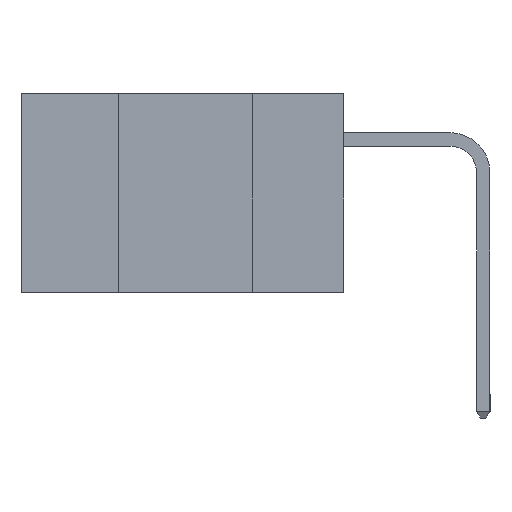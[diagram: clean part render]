
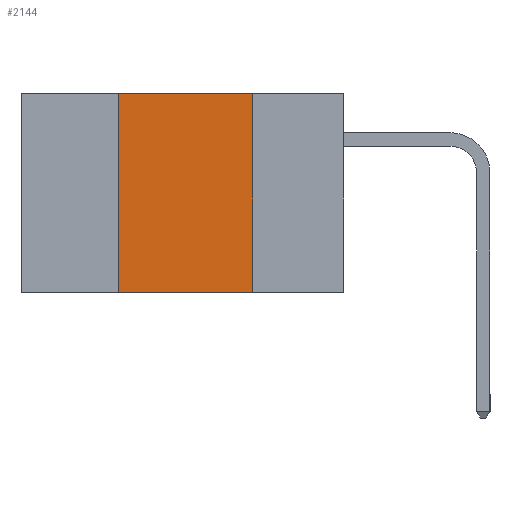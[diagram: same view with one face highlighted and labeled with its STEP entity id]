
A CAD part, left-side view. The second image highlights one B-rep face of the part: STEP entity #2144.
In plain terms, the highlighted planar face has unit normal (-1, 0, 0).
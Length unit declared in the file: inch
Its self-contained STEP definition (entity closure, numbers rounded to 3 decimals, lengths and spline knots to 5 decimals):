
#151 = EDGE_CURVE ( 'NONE', #18014, #11505, #10872, .T. ) ;
#983 = VERTEX_POINT ( 'NONE', #18293 ) ;
#1984 = CARTESIAN_POINT ( 'NONE',  ( 0., 0.17, -0.37 ) ) ;
#2144 = ADVANCED_FACE ( 'NONE', ( #19968 ), #10335, .F. ) ;
#2215 = ORIENTED_EDGE ( 'NONE', *, *, #21178, .F. ) ;
#4227 = CARTESIAN_POINT ( 'NONE',  ( 0., 0.17, -0.37 ) ) ;
#4816 = VERTEX_POINT ( 'NONE', #19660 ) ;
#5437 = VECTOR ( 'NONE', #21842, 39.37008 ) ;
#6388 = ORIENTED_EDGE ( 'NONE', *, *, #16742, .F. ) ;
#8524 = DIRECTION ( 'NONE',  ( 1., 0., 0. ) ) ;
#8575 = DIRECTION ( 'NONE',  ( 0., 0., -1. ) ) ;
#9045 = CARTESIAN_POINT ( 'NONE',  ( 0., 0.6, 0. ) ) ;
#9457 = VECTOR ( 'NONE', #14872, 39.37008 ) ;
#9510 = CARTESIAN_POINT ( 'NONE',  ( 0., 0.17, 0. ) ) ;
#9820 = AXIS2_PLACEMENT_3D ( 'NONE', #9045, #8524, #8575 ) ;
#10335 = PLANE ( 'NONE',  #9820 ) ;
#10872 = LINE ( 'NONE', #4227, #19280 ) ;
#11433 = CARTESIAN_POINT ( 'NONE',  ( 0., 0.6, 0. ) ) ;
#11505 = VERTEX_POINT ( 'NONE', #1984 ) ;
#11613 = DIRECTION ( 'NONE',  ( 0., 0., -1. ) ) ;
#13068 = ORIENTED_EDGE ( 'NONE', *, *, #151, .F. ) ;
#13365 = EDGE_CURVE ( 'NONE', #983, #11505, #13457, .T. ) ;
#13457 = LINE ( 'NONE', #20928, #21269 ) ;
#13500 = EDGE_LOOP ( 'NONE', ( #13068, #2215, #6388, #19386 ) ) ;
#13821 = LINE ( 'NONE', #21730, #5437 ) ;
#13923 = LINE ( 'NONE', #11433, #9457 ) ;
#14872 = DIRECTION ( 'NONE',  ( 0., -1., 0. ) ) ;
#16742 = EDGE_CURVE ( 'NONE', #983, #4816, #13821, .T. ) ;
#18014 = VERTEX_POINT ( 'NONE', #9510 ) ;
#18293 = CARTESIAN_POINT ( 'NONE',  ( 0., 0.42, -0.37 ) ) ;
#19280 = VECTOR ( 'NONE', #11613, 39.37008 ) ;
#19386 = ORIENTED_EDGE ( 'NONE', *, *, #13365, .T. ) ;
#19660 = CARTESIAN_POINT ( 'NONE',  ( 0., 0.42, 0. ) ) ;
#19968 = FACE_OUTER_BOUND ( 'NONE', #13500, .T. ) ;
#20928 = CARTESIAN_POINT ( 'NONE',  ( 0., 0.6, -0.37 ) ) ;
#21025 = DIRECTION ( 'NONE',  ( 0., -1., 0. ) ) ;
#21178 = EDGE_CURVE ( 'NONE', #4816, #18014, #13923, .T. ) ;
#21269 = VECTOR ( 'NONE', #21025, 39.37008 ) ;
#21730 = CARTESIAN_POINT ( 'NONE',  ( 0., 0.42, -0.37 ) ) ;
#21842 = DIRECTION ( 'NONE',  ( 0., 0., 1. ) ) ;
